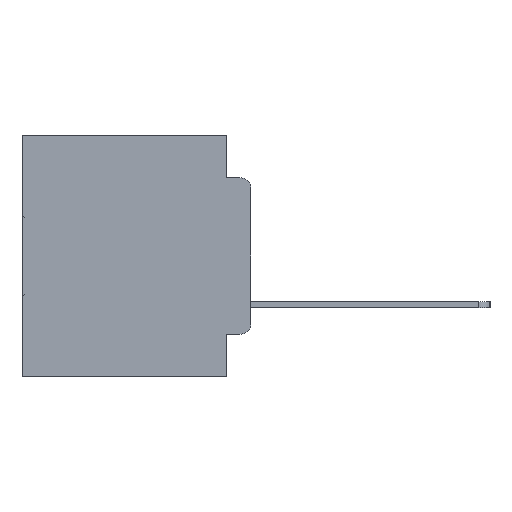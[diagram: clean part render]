
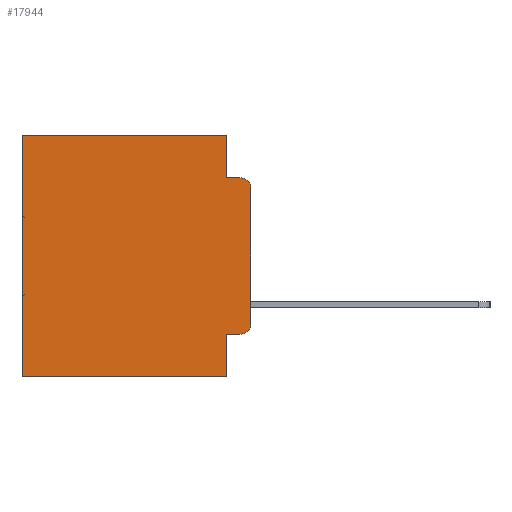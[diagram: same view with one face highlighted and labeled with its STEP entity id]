
A CAD part, left-side view. The second image highlights one B-rep face of the part: STEP entity #17944.
In plain terms, the highlighted planar face has unit normal (-1, 0, 0).
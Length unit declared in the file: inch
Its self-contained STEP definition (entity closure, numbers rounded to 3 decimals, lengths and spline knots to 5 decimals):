
#916 = CARTESIAN_POINT ( 'NONE',  ( 0.298, 0.473, 0. ) ) ;
#993 = CARTESIAN_POINT ( 'NONE',  ( 0.298, 0., -0.3915 ) ) ;
#1377 = ORIENTED_EDGE ( 'NONE', *, *, #33057, .F. ) ;
#2324 = DIRECTION ( 'NONE',  ( 0., 0., -1. ) ) ;
#2841 = CARTESIAN_POINT ( 'NONE',  ( 0.298, 0.051, -0.0885 ) ) ;
#3074 = DIRECTION ( 'NONE',  ( 1., 0., 0. ) ) ;
#3576 = VERTEX_POINT ( 'NONE', #27202 ) ;
#3937 = VECTOR ( 'NONE', #31869, 39.37008 ) ;
#4006 = ORIENTED_EDGE ( 'NONE', *, *, #31334, .T. ) ;
#4442 = VECTOR ( 'NONE', #10142, 39.37008 ) ;
#4651 = DIRECTION ( 'NONE',  ( 0., -1., 0. ) ) ;
#4808 = CARTESIAN_POINT ( 'NONE',  ( 0.298, 0.051, -0.5 ) ) ;
#4853 = LINE ( 'NONE', #16582, #33373 ) ;
#5069 = EDGE_LOOP ( 'NONE', ( #25620, #5714, #20300, #28900, #25216, #33796, #20725, #1377, #4006, #5755 ) ) ;
#5249 = VECTOR ( 'NONE', #4651, 39.37008 ) ;
#5628 = CARTESIAN_POINT ( 'NONE',  ( 0.298, 0.02, -0.3915 ) ) ;
#5714 = ORIENTED_EDGE ( 'NONE', *, *, #20156, .T. ) ;
#5755 = ORIENTED_EDGE ( 'NONE', *, *, #22560, .T. ) ;
#6142 = DIRECTION ( 'NONE',  ( 0., 1., 0. ) ) ;
#7117 = EDGE_CURVE ( 'NONE', #13197, #31247, #11719, .T. ) ;
#7177 = CARTESIAN_POINT ( 'NONE',  ( 0.298, 0., -0.5 ) ) ;
#7327 = EDGE_CURVE ( 'NONE', #15460, #19672, #4853, .T. ) ;
#8343 = VECTOR ( 'NONE', #20186, 39.37008 ) ;
#8432 = DIRECTION ( 'NONE',  ( 0., 0., -1. ) ) ;
#9155 = EDGE_CURVE ( 'NONE', #19672, #25038, #16359, .T. ) ;
#9797 = AXIS2_PLACEMENT_3D ( 'NONE', #5628, #24599, #8432 ) ;
#10142 = DIRECTION ( 'NONE',  ( 0., 1., 0. ) ) ;
#10168 = CARTESIAN_POINT ( 'NONE',  ( 0.298, 0.051, 0. ) ) ;
#10382 = VERTEX_POINT ( 'NONE', #29435 ) ;
#10687 = LINE ( 'NONE', #10168, #31994 ) ;
#10952 = VERTEX_POINT ( 'NONE', #21902 ) ;
#11236 = LINE ( 'NONE', #23992, #3937 ) ;
#11719 = LINE ( 'NONE', #7177, #4442 ) ;
#12029 = CARTESIAN_POINT ( 'NONE',  ( 0.298, 0.02, -0.0885 ) ) ;
#13197 = VERTEX_POINT ( 'NONE', #4808 ) ;
#13452 = CIRCLE ( 'NONE', #9797, 0.02 ) ;
#13475 = LINE ( 'NONE', #22425, #33854 ) ;
#13600 = DIRECTION ( 'NONE',  ( 0., -1., 0. ) ) ;
#13972 = CARTESIAN_POINT ( 'NONE',  ( 0.298, 0., 0. ) ) ;
#15460 = VERTEX_POINT ( 'NONE', #30492 ) ;
#15583 = LINE ( 'NONE', #916, #8343 ) ;
#15657 = DIRECTION ( 'NONE',  ( 0., 0., -1. ) ) ;
#16359 = LINE ( 'NONE', #32229, #29638 ) ;
#16582 = CARTESIAN_POINT ( 'NONE',  ( 0.298, 0.051, 0. ) ) ;
#17944 = ADVANCED_FACE ( 'NONE', ( #29182 ), #19560, .F. ) ;
#18352 = CARTESIAN_POINT ( 'NONE',  ( 0.298, 0.051, -0.4115 ) ) ;
#18808 = DIRECTION ( 'NONE',  ( -1., 0., 0. ) ) ;
#19017 = LINE ( 'NONE', #18352, #5249 ) ;
#19560 = PLANE ( 'NONE',  #20041 ) ;
#19672 = VERTEX_POINT ( 'NONE', #2841 ) ;
#20041 = AXIS2_PLACEMENT_3D ( 'NONE', #13972, #3074, #22191 ) ;
#20156 = EDGE_CURVE ( 'NONE', #30193, #25038, #22873, .T. ) ;
#20186 = DIRECTION ( 'NONE',  ( 0., 0., -1. ) ) ;
#20300 = ORIENTED_EDGE ( 'NONE', *, *, #9155, .F. ) ;
#20725 = ORIENTED_EDGE ( 'NONE', *, *, #7117, .F. ) ;
#21468 = CARTESIAN_POINT ( 'NONE',  ( 0.298, 0., -0.1085 ) ) ;
#21507 = EDGE_CURVE ( 'NONE', #15460, #10952, #13475, .T. ) ;
#21902 = CARTESIAN_POINT ( 'NONE',  ( 0.298, 0.473, 0. ) ) ;
#22191 = DIRECTION ( 'NONE',  ( 0., 0., -1. ) ) ;
#22425 = CARTESIAN_POINT ( 'NONE',  ( 0.298, 0., 0. ) ) ;
#22560 = EDGE_CURVE ( 'NONE', #3576, #29363, #13452, .T. ) ;
#22873 = CIRCLE ( 'NONE', #26009, 0.02 ) ;
#23674 = EDGE_CURVE ( 'NONE', #30193, #29363, #11236, .T. ) ;
#23992 = CARTESIAN_POINT ( 'NONE',  ( 0.298, 0., 0. ) ) ;
#24599 = DIRECTION ( 'NONE',  ( -1., 0., 0. ) ) ;
#25038 = VERTEX_POINT ( 'NONE', #12029 ) ;
#25216 = ORIENTED_EDGE ( 'NONE', *, *, #21507, .T. ) ;
#25620 = ORIENTED_EDGE ( 'NONE', *, *, #23674, .F. ) ;
#26009 = AXIS2_PLACEMENT_3D ( 'NONE', #34514, #18808, #2324 ) ;
#27171 = DIRECTION ( 'NONE',  ( 0., 0., -1. ) ) ;
#27202 = CARTESIAN_POINT ( 'NONE',  ( 0.298, 0.02, -0.4115 ) ) ;
#28900 = ORIENTED_EDGE ( 'NONE', *, *, #7327, .F. ) ;
#29182 = FACE_OUTER_BOUND ( 'NONE', #5069, .T. ) ;
#29363 = VERTEX_POINT ( 'NONE', #993 ) ;
#29435 = CARTESIAN_POINT ( 'NONE',  ( 0.298, 0.051, -0.4115 ) ) ;
#29638 = VECTOR ( 'NONE', #13600, 39.37008 ) ;
#30193 = VERTEX_POINT ( 'NONE', #21468 ) ;
#30492 = CARTESIAN_POINT ( 'NONE',  ( 0.298, 0.051, 0. ) ) ;
#31230 = CARTESIAN_POINT ( 'NONE',  ( 0.298, 0.473, -0.5 ) ) ;
#31247 = VERTEX_POINT ( 'NONE', #31230 ) ;
#31334 = EDGE_CURVE ( 'NONE', #10382, #3576, #19017, .T. ) ;
#31869 = DIRECTION ( 'NONE',  ( 0., 0., -1. ) ) ;
#31994 = VECTOR ( 'NONE', #15657, 39.37008 ) ;
#32229 = CARTESIAN_POINT ( 'NONE',  ( 0.298, 0.051, -0.0885 ) ) ;
#33057 = EDGE_CURVE ( 'NONE', #10382, #13197, #10687, .T. ) ;
#33373 = VECTOR ( 'NONE', #27171, 39.37008 ) ;
#33796 = ORIENTED_EDGE ( 'NONE', *, *, #34822, .T. ) ;
#33854 = VECTOR ( 'NONE', #6142, 39.37008 ) ;
#34514 = CARTESIAN_POINT ( 'NONE',  ( 0.298, 0.02, -0.1085 ) ) ;
#34822 = EDGE_CURVE ( 'NONE', #10952, #31247, #15583, .T. ) ;
